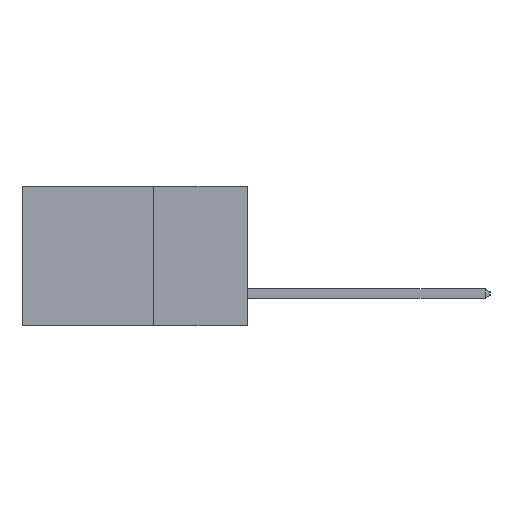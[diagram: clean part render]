
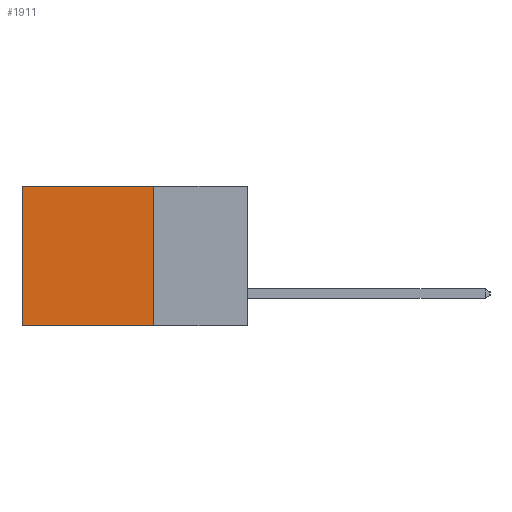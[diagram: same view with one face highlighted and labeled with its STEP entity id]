
A CAD part, left-side view. The second image highlights one B-rep face of the part: STEP entity #1911.
In plain terms, the highlighted planar face has unit normal (-1, 0, 0).
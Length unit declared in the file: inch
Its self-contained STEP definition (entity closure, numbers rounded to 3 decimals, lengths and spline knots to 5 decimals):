
#129 = ORIENTED_EDGE ( 'NONE', *, *, #3784, .F. ) ;
#250 = DIRECTION ( 'NONE',  ( 0., 0., -1. ) ) ;
#256 = DIRECTION ( 'NONE',  ( 1., 0., 0. ) ) ;
#344 = EDGE_CURVE ( 'NONE', #7870, #3571, #6581, .T. ) ;
#353 = PLANE ( 'NONE',  #5312 ) ;
#740 = VECTOR ( 'NONE', #9840, 39.37008 ) ;
#929 = CARTESIAN_POINT ( 'NONE',  ( 0.2615, 0.25, -0.37 ) ) ;
#1533 = VECTOR ( 'NONE', #6881, 39.37008 ) ;
#1911 = ADVANCED_FACE ( 'NONE', ( #2531 ), #353, .F. ) ;
#2253 = VERTEX_POINT ( 'NONE', #3465 ) ;
#2531 = FACE_OUTER_BOUND ( 'NONE', #9230, .T. ) ;
#2596 = VECTOR ( 'NONE', #3020, 39.37008 ) ;
#2605 = ORIENTED_EDGE ( 'NONE', *, *, #344, .F. ) ;
#3020 = DIRECTION ( 'NONE',  ( 0., 0., -1. ) ) ;
#3199 = LINE ( 'NONE', #10462, #2596 ) ;
#3465 = CARTESIAN_POINT ( 'NONE',  ( 0.2615, 0.6, -0.37 ) ) ;
#3571 = VERTEX_POINT ( 'NONE', #9348 ) ;
#3712 = CARTESIAN_POINT ( 'NONE',  ( 0.2615, 0.25, 0. ) ) ;
#3784 = EDGE_CURVE ( 'NONE', #3571, #2253, #5766, .T. ) ;
#5019 = EDGE_CURVE ( 'NONE', #7870, #10064, #7178, .T. ) ;
#5197 = EDGE_CURVE ( 'NONE', #10064, #2253, #3199, .T. ) ;
#5312 = AXIS2_PLACEMENT_3D ( 'NONE', #929, #256, #250 ) ;
#5766 = LINE ( 'NONE', #9852, #740 ) ;
#6458 = CARTESIAN_POINT ( 'NONE',  ( 0.2615, 0.25, -0.37 ) ) ;
#6581 = LINE ( 'NONE', #6458, #1533 ) ;
#6881 = DIRECTION ( 'NONE',  ( 0., 0., -1. ) ) ;
#7027 = CARTESIAN_POINT ( 'NONE',  ( 0.2615, 0.6, 0. ) ) ;
#7178 = LINE ( 'NONE', #8424, #11709 ) ;
#7870 = VERTEX_POINT ( 'NONE', #3712 ) ;
#8424 = CARTESIAN_POINT ( 'NONE',  ( 0.2615, 0.25, 0. ) ) ;
#9230 = EDGE_LOOP ( 'NONE', ( #11899, #129, #2605, #9420 ) ) ;
#9328 = DIRECTION ( 'NONE',  ( 0., 1., 0. ) ) ;
#9348 = CARTESIAN_POINT ( 'NONE',  ( 0.2615, 0.25, -0.37 ) ) ;
#9420 = ORIENTED_EDGE ( 'NONE', *, *, #5019, .T. ) ;
#9840 = DIRECTION ( 'NONE',  ( 0., 1., 0. ) ) ;
#9852 = CARTESIAN_POINT ( 'NONE',  ( 0.2615, 0.25, -0.37 ) ) ;
#10064 = VERTEX_POINT ( 'NONE', #7027 ) ;
#10462 = CARTESIAN_POINT ( 'NONE',  ( 0.2615, 0.6, -0.37 ) ) ;
#11709 = VECTOR ( 'NONE', #9328, 39.37008 ) ;
#11899 = ORIENTED_EDGE ( 'NONE', *, *, #5197, .T. ) ;
